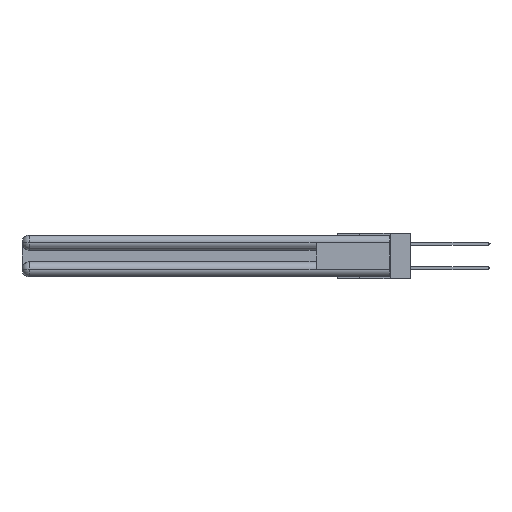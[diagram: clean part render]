
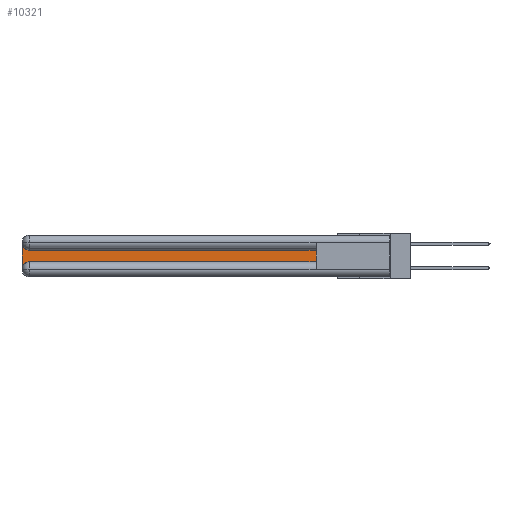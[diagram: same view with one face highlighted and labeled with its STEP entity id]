
A CAD part, left-side view. The second image highlights one B-rep face of the part: STEP entity #10321.
In plain terms, the highlighted planar face has unit normal (-1, 0, 0).
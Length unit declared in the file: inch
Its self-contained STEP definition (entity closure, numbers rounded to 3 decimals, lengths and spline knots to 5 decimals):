
#324 = ORIENTED_EDGE ( 'NONE', *, *, #32107, .T. ) ;
#595 = EDGE_CURVE ( 'NONE', #21601, #27926, #6817, .T. ) ;
#1113 = CARTESIAN_POINT ( 'NONE',  ( 0.075, 0.6, -0.2175 ) ) ;
#1373 = LINE ( 'NONE', #21526, #3327 ) ;
#2198 = VERTEX_POINT ( 'NONE', #16590 ) ;
#3327 = VECTOR ( 'NONE', #16627, 39.37008 ) ;
#3925 = VERTEX_POINT ( 'NONE', #23743 ) ;
#3994 = AXIS2_PLACEMENT_3D ( 'NONE', #12392, #30065, #15221 ) ;
#5755 = LINE ( 'NONE', #20160, #9624 ) ;
#6328 = AXIS2_PLACEMENT_3D ( 'NONE', #32128, #26972, #17394 ) ;
#6817 = CIRCLE ( 'NONE', #3994, 0.06 ) ;
#9504 = CIRCLE ( 'NONE', #6328, 0.06 ) ;
#9624 = VECTOR ( 'NONE', #25371, 39.37008 ) ;
#9743 = ORIENTED_EDGE ( 'NONE', *, *, #29727, .T. ) ;
#9824 = EDGE_CURVE ( 'NONE', #10172, #28570, #1373, .T. ) ;
#10172 = VERTEX_POINT ( 'NONE', #16867 ) ;
#10276 = FACE_OUTER_BOUND ( 'NONE', #26006, .T. ) ;
#10321 = ADVANCED_FACE ( 'NONE', ( #10276 ), #13915, .F. ) ;
#11938 = ORIENTED_EDGE ( 'NONE', *, *, #595, .T. ) ;
#12214 = LINE ( 'NONE', #29740, #17248 ) ;
#12392 = CARTESIAN_POINT ( 'NONE',  ( 0.075, 2.94, -0.2775 ) ) ;
#13915 = PLANE ( 'NONE',  #14856 ) ;
#14034 = DIRECTION ( 'NONE',  ( 1., 0., 0. ) ) ;
#14639 = ORIENTED_EDGE ( 'NONE', *, *, #9824, .T. ) ;
#14856 = AXIS2_PLACEMENT_3D ( 'NONE', #29034, #14034, #31372 ) ;
#14869 = DIRECTION ( 'NONE',  ( 0., 1., 0. ) ) ;
#15221 = DIRECTION ( 'NONE',  ( 0., 0., -1. ) ) ;
#16590 = CARTESIAN_POINT ( 'NONE',  ( 0.075, 3., -0.0625 ) ) ;
#16627 = DIRECTION ( 'NONE',  ( 0., 0., 1. ) ) ;
#16867 = CARTESIAN_POINT ( 'NONE',  ( 0.075, 0.6, -0.2175 ) ) ;
#17248 = VECTOR ( 'NONE', #14869, 39.37008 ) ;
#17394 = DIRECTION ( 'NONE',  ( 0., 0., -1. ) ) ;
#17553 = LINE ( 'NONE', #1113, #19100 ) ;
#18515 = DIRECTION ( 'NONE',  ( 0., -1., 0. ) ) ;
#18677 = CARTESIAN_POINT ( 'NONE',  ( 0.075, 0.6, -0.1225 ) ) ;
#19100 = VECTOR ( 'NONE', #18515, 39.37008 ) ;
#19925 = ORIENTED_EDGE ( 'NONE', *, *, #27855, .T. ) ;
#20160 = CARTESIAN_POINT ( 'NONE',  ( 0.075, 3., -0.2175 ) ) ;
#20265 = CARTESIAN_POINT ( 'NONE',  ( 0.075, 2.94, -0.2175 ) ) ;
#21526 = CARTESIAN_POINT ( 'NONE',  ( 0.075, 0.6, -0.2175 ) ) ;
#21601 = VERTEX_POINT ( 'NONE', #21740 ) ;
#21740 = CARTESIAN_POINT ( 'NONE',  ( 0.075, 3., -0.2775 ) ) ;
#23743 = CARTESIAN_POINT ( 'NONE',  ( 0.075, 2.94, -0.1225 ) ) ;
#25371 = DIRECTION ( 'NONE',  ( 0., 0., -1. ) ) ;
#26006 = EDGE_LOOP ( 'NONE', ( #26980, #9743, #19925, #11938, #324, #14639 ) ) ;
#26972 = DIRECTION ( 'NONE',  ( 1., 0., 0. ) ) ;
#26980 = ORIENTED_EDGE ( 'NONE', *, *, #30349, .T. ) ;
#27855 = EDGE_CURVE ( 'NONE', #2198, #21601, #5755, .T. ) ;
#27926 = VERTEX_POINT ( 'NONE', #20265 ) ;
#28570 = VERTEX_POINT ( 'NONE', #18677 ) ;
#29034 = CARTESIAN_POINT ( 'NONE',  ( 0.075, 3., -0.1225 ) ) ;
#29727 = EDGE_CURVE ( 'NONE', #3925, #2198, #9504, .T. ) ;
#29740 = CARTESIAN_POINT ( 'NONE',  ( 0.075, 0.6, -0.1225 ) ) ;
#30065 = DIRECTION ( 'NONE',  ( 1., 0., 0. ) ) ;
#30349 = EDGE_CURVE ( 'NONE', #28570, #3925, #12214, .T. ) ;
#31372 = DIRECTION ( 'NONE',  ( 0., 0., -1. ) ) ;
#32107 = EDGE_CURVE ( 'NONE', #27926, #10172, #17553, .T. ) ;
#32128 = CARTESIAN_POINT ( 'NONE',  ( 0.075, 2.94, -0.0625 ) ) ;
